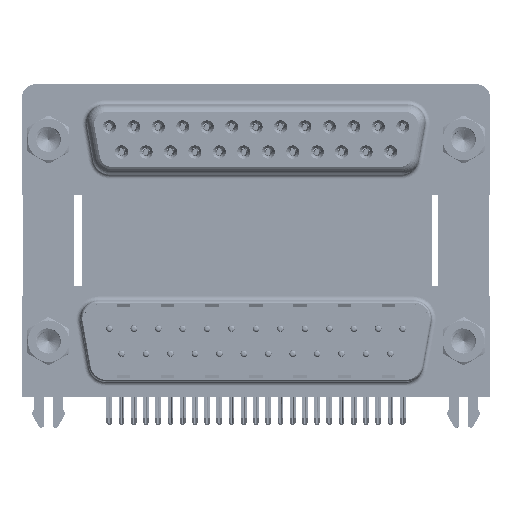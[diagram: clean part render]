
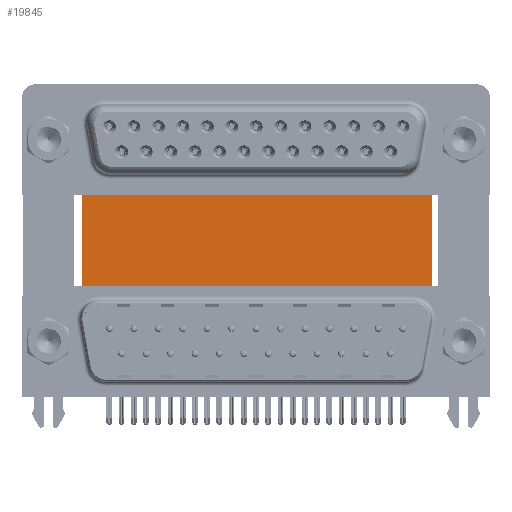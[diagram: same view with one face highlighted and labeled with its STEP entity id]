
A CAD part, top view. The second image highlights one B-rep face of the part: STEP entity #19845.
In plain terms, the highlighted planar face has unit normal (0, 0, 1).
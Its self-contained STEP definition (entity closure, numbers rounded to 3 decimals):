
#1748 = CARTESIAN_POINT ( 'NONE',  ( 43.43, -3.735, -12. ) ) ;
#4464 = VECTOR ( 'NONE', #40365, 1000. ) ;
#6670 = DIRECTION ( 'NONE',  ( 0., -1., 0. ) ) ;
#6975 = CARTESIAN_POINT ( 'NONE',  ( 3.79, 16.585, -12. ) ) ;
#8088 = DIRECTION ( 'NONE',  ( 0., 0., -1. ) ) ;
#8510 = AXIS2_PLACEMENT_3D ( 'NONE', #40211, #8088, #55132 ) ;
#8543 = CARTESIAN_POINT ( 'NONE',  ( 43.43, 16.585, -12. ) ) ;
#10588 = ORIENTED_EDGE ( 'NONE', *, *, #26623, .T. ) ;
#11058 = LINE ( 'NONE', #21349, #4464 ) ;
#11105 = EDGE_LOOP ( 'NONE', ( #20582, #55381, #32428, #10588 ) ) ;
#11860 = LINE ( 'NONE', #45825, #44308 ) ;
#15490 = CARTESIAN_POINT ( 'NONE',  ( 3.79, 16.585, -12. ) ) ;
#19845 = ADVANCED_FACE ( 'NONE', ( #22126 ), #31806, .F. ) ;
#20582 = ORIENTED_EDGE ( 'NONE', *, *, #58323, .T. ) ;
#21349 = CARTESIAN_POINT ( 'NONE',  ( 43.43, 16.585, -12. ) ) ;
#22126 = FACE_OUTER_BOUND ( 'NONE', #11105, .T. ) ;
#25347 = VERTEX_POINT ( 'NONE', #15490 ) ;
#26026 = VERTEX_POINT ( 'NONE', #1748 ) ;
#26182 = VECTOR ( 'NONE', #6670, 1000. ) ;
#26623 = EDGE_CURVE ( 'NONE', #25347, #34770, #40666, .T. ) ;
#28696 = EDGE_CURVE ( 'NONE', #42158, #26026, #11058, .T. ) ;
#30890 = EDGE_CURVE ( 'NONE', #25347, #42158, #11860, .T. ) ;
#31806 = PLANE ( 'NONE',  #8510 ) ;
#32428 = ORIENTED_EDGE ( 'NONE', *, *, #30890, .F. ) ;
#34770 = VERTEX_POINT ( 'NONE', #41933 ) ;
#35485 = VECTOR ( 'NONE', #54579, 1000. ) ;
#40211 = CARTESIAN_POINT ( 'NONE',  ( 3.79, 16.585, -12. ) ) ;
#40365 = DIRECTION ( 'NONE',  ( 0., -1., 0. ) ) ;
#40666 = LINE ( 'NONE', #6975, #26182 ) ;
#41933 = CARTESIAN_POINT ( 'NONE',  ( 3.79, -3.735, -12. ) ) ;
#42158 = VERTEX_POINT ( 'NONE', #8543 ) ;
#44308 = VECTOR ( 'NONE', #59522, 1000. ) ;
#45825 = CARTESIAN_POINT ( 'NONE',  ( 3.79, 16.585, -12. ) ) ;
#46167 = LINE ( 'NONE', #46474, #35485 ) ;
#46474 = CARTESIAN_POINT ( 'NONE',  ( 3.79, -3.735, -12. ) ) ;
#54579 = DIRECTION ( 'NONE',  ( 1., 0., 0. ) ) ;
#55132 = DIRECTION ( 'NONE',  ( -1., 0., 0. ) ) ;
#55381 = ORIENTED_EDGE ( 'NONE', *, *, #28696, .F. ) ;
#58323 = EDGE_CURVE ( 'NONE', #34770, #26026, #46167, .T. ) ;
#59522 = DIRECTION ( 'NONE',  ( 1., 0., 0. ) ) ;
